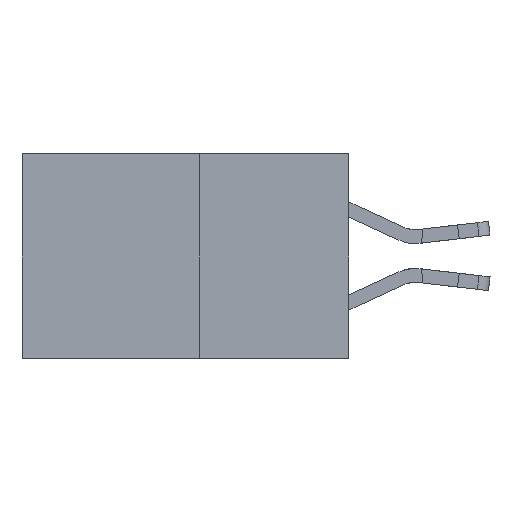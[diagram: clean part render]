
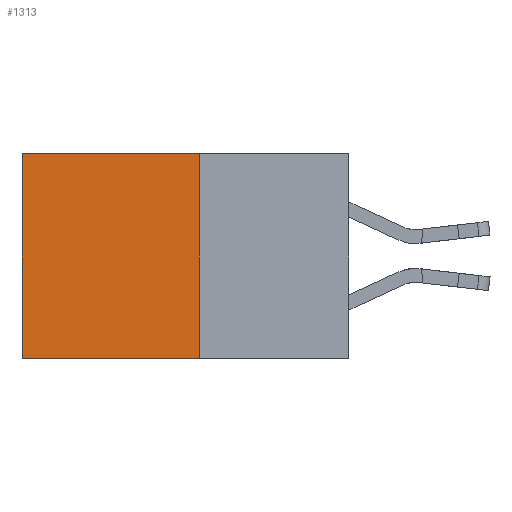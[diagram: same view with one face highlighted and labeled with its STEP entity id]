
A CAD part, left-side view. The second image highlights one B-rep face of the part: STEP entity #1313.
In plain terms, the highlighted planar face has unit normal (-1, 0, 0).
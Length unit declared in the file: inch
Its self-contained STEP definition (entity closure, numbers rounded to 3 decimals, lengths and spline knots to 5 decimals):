
#472 = EDGE_CURVE ( 'NONE', #3215, #12575, #13998, .T. ) ;
#1258 = VECTOR ( 'NONE', #19811, 39.37008 ) ;
#1313 = ADVANCED_FACE ( 'NONE', ( #16216 ), #17093, .F. ) ;
#2272 = CARTESIAN_POINT ( 'NONE',  ( 0.277, 0.59, -0.37 ) ) ;
#3141 = VERTEX_POINT ( 'NONE', #24808 ) ;
#3215 = VERTEX_POINT ( 'NONE', #14876 ) ;
#4933 = DIRECTION ( 'NONE',  ( 0., 0., -1. ) ) ;
#5518 = CARTESIAN_POINT ( 'NONE',  ( 0.277, 0.59, -0.37 ) ) ;
#5896 = DIRECTION ( 'NONE',  ( 1., 0., 0. ) ) ;
#5990 = ORIENTED_EDGE ( 'NONE', *, *, #18627, .T. ) ;
#6011 = DIRECTION ( 'NONE',  ( 0., 1., 0. ) ) ;
#8287 = ORIENTED_EDGE ( 'NONE', *, *, #472, .T. ) ;
#9785 = VECTOR ( 'NONE', #4933, 39.37008 ) ;
#10667 = CARTESIAN_POINT ( 'NONE',  ( 0.277, 0.27, -0.37 ) ) ;
#10723 = DIRECTION ( 'NONE',  ( 0., 0., -1. ) ) ;
#11715 = LINE ( 'NONE', #17835, #1258 ) ;
#12441 = EDGE_LOOP ( 'NONE', ( #8287, #23006, #19884, #5990 ) ) ;
#12575 = VERTEX_POINT ( 'NONE', #5518 ) ;
#13998 = LINE ( 'NONE', #2272, #9785 ) ;
#14876 = CARTESIAN_POINT ( 'NONE',  ( 0.277, 0.59, 0. ) ) ;
#15925 = CARTESIAN_POINT ( 'NONE',  ( 0.277, 0.27, -0.37 ) ) ;
#16216 = FACE_OUTER_BOUND ( 'NONE', #12441, .T. ) ;
#16325 = CARTESIAN_POINT ( 'NONE',  ( 0.277, 0.27, -0.37 ) ) ;
#17093 = PLANE ( 'NONE',  #23683 ) ;
#17566 = EDGE_CURVE ( 'NONE', #17618, #3141, #24586, .T. ) ;
#17618 = VERTEX_POINT ( 'NONE', #22497 ) ;
#17835 = CARTESIAN_POINT ( 'NONE',  ( 0.277, 0.27, 0. ) ) ;
#18428 = VECTOR ( 'NONE', #6011, 39.37008 ) ;
#18627 = EDGE_CURVE ( 'NONE', #17618, #3215, #11715, .T. ) ;
#19811 = DIRECTION ( 'NONE',  ( 0., 1., 0. ) ) ;
#19884 = ORIENTED_EDGE ( 'NONE', *, *, #17566, .F. ) ;
#20062 = VECTOR ( 'NONE', #24329, 39.37008 ) ;
#20342 = EDGE_CURVE ( 'NONE', #3141, #12575, #24195, .T. ) ;
#22497 = CARTESIAN_POINT ( 'NONE',  ( 0.277, 0.27, 0. ) ) ;
#23006 = ORIENTED_EDGE ( 'NONE', *, *, #20342, .F. ) ;
#23683 = AXIS2_PLACEMENT_3D ( 'NONE', #16325, #5896, #10723 ) ;
#24195 = LINE ( 'NONE', #15925, #18428 ) ;
#24329 = DIRECTION ( 'NONE',  ( 0., 0., -1. ) ) ;
#24586 = LINE ( 'NONE', #10667, #20062 ) ;
#24808 = CARTESIAN_POINT ( 'NONE',  ( 0.277, 0.27, -0.37 ) ) ;
